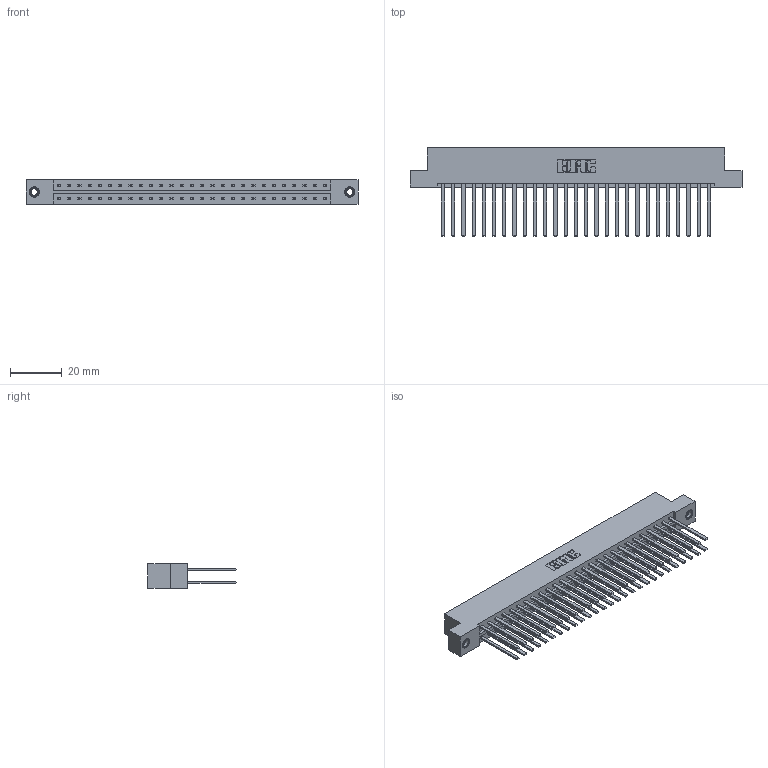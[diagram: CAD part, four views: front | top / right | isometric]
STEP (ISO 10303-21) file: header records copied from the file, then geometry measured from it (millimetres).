
FILE_DESCRIPTION (( 'STEP AP203' ), '1' );
FILE_NAME ('833-054-544-207.STEP', '2020-06-04T21:15:49', ( '' ), ( '' ), 'SwSTEP 2.0', 'SolidWorks 2020', '' );
FILE_SCHEMA (( 'CONFIG_CONTROL_DESIGN' ));
Length unit declared in the file: inch
Products named in the file (4): 833-054-544-207; 833 Part_Flush - .156 Dia - TI; 345-292-001_345-293-144; 345-250-001_345-250-005-103
Assembly tree (57 placements, depth 2):
  833-054-544-207
    833 Part_Flush - .156 Dia - TI
    345-292-001_345-293-144  x54
    345-250-001_345-250-005-103  x2
Bounding box: 128.52 x 34.3 x 9.4 mm (x, y, z)
Volume: 13724.8 mm3; surface area: 18536.3 mm2
Topology: 57 solids, 57 shells, 2658 faces, 7845 edges, 5150 vertices
Faces by surface type: plane 1830, cylinder 812, cone 12, torus 4
Entity records: 20312 total; most frequent: CARTESIAN_POINT 3365, ORIENTED_EDGE 3294, DIRECTION 2929, EDGE_CURVE 1647, VECTOR 1503, LINE 1503, VERTEX_POINT 1092, AXIS2_PLACEMENT_3D 713
